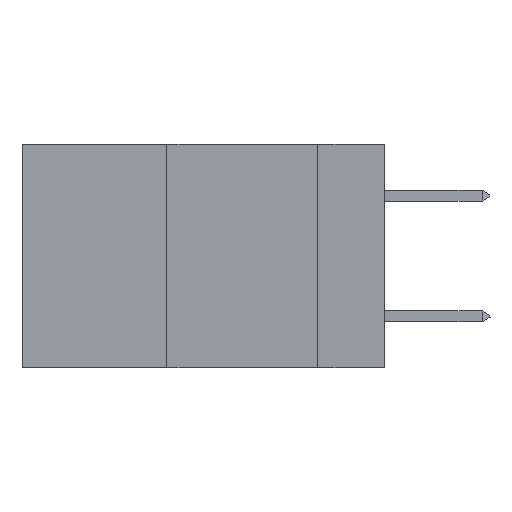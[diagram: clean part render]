
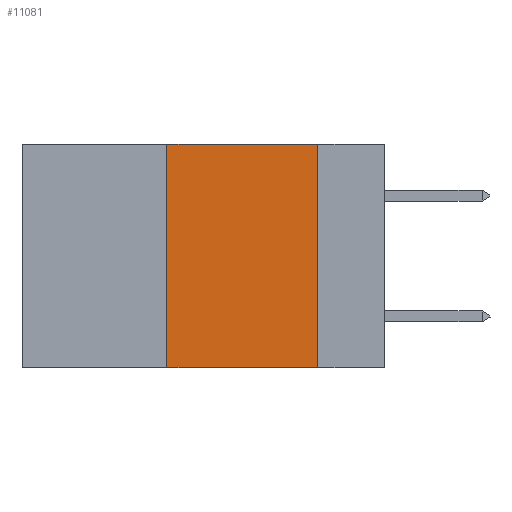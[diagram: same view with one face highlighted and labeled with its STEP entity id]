
A CAD part, left-side view. The second image highlights one B-rep face of the part: STEP entity #11081.
In plain terms, the highlighted planar face has unit normal (-1, 0, 0).
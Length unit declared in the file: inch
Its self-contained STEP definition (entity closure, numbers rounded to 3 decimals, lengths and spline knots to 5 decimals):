
#957 = DIRECTION ( 'NONE',  ( 0., 0., -1. ) ) ;
#1216 = EDGE_LOOP ( 'NONE', ( #5683, #15157, #14029, #14795 ) ) ;
#2191 = VECTOR ( 'NONE', #5154, 39.37008 ) ;
#2576 = CARTESIAN_POINT ( 'NONE',  ( 0., 0.36, 0. ) ) ;
#3693 = EDGE_CURVE ( 'NONE', #4525, #5397, #11834, .T. ) ;
#3724 = CARTESIAN_POINT ( 'NONE',  ( 0., 0.11, -0.37 ) ) ;
#4525 = VERTEX_POINT ( 'NONE', #11660 ) ;
#5057 = EDGE_CURVE ( 'NONE', #7020, #4525, #5782, .T. ) ;
#5154 = DIRECTION ( 'NONE',  ( 0., -1., 0. ) ) ;
#5188 = DIRECTION ( 'NONE',  ( 0., 0., -1. ) ) ;
#5397 = VERTEX_POINT ( 'NONE', #7984 ) ;
#5683 = ORIENTED_EDGE ( 'NONE', *, *, #15193, .F. ) ;
#5745 = VERTEX_POINT ( 'NONE', #3724 ) ;
#5782 = LINE ( 'NONE', #2576, #12210 ) ;
#6328 = LINE ( 'NONE', #12430, #12754 ) ;
#6542 = LINE ( 'NONE', #11416, #11831 ) ;
#6991 = PLANE ( 'NONE',  #10068 ) ;
#7020 = VERTEX_POINT ( 'NONE', #15474 ) ;
#7984 = CARTESIAN_POINT ( 'NONE',  ( 0., 0.11, 0. ) ) ;
#8208 = DIRECTION ( 'NONE',  ( 1., 0., 0. ) ) ;
#9225 = FACE_OUTER_BOUND ( 'NONE', #1216, .T. ) ;
#10068 = AXIS2_PLACEMENT_3D ( 'NONE', #15449, #8208, #957 ) ;
#11046 = DIRECTION ( 'NONE',  ( 0., 0., 1. ) ) ;
#11081 = ADVANCED_FACE ( 'NONE', ( #9225 ), #6991, .F. ) ;
#11416 = CARTESIAN_POINT ( 'NONE',  ( 0., 0.6, -0.37 ) ) ;
#11660 = CARTESIAN_POINT ( 'NONE',  ( 0., 0.36, 0. ) ) ;
#11831 = VECTOR ( 'NONE', #12615, 39.37008 ) ;
#11834 = LINE ( 'NONE', #13589, #2191 ) ;
#12210 = VECTOR ( 'NONE', #11046, 39.37008 ) ;
#12430 = CARTESIAN_POINT ( 'NONE',  ( 0., 0.11, 0. ) ) ;
#12615 = DIRECTION ( 'NONE',  ( 0., -1., 0. ) ) ;
#12754 = VECTOR ( 'NONE', #5188, 39.37008 ) ;
#13589 = CARTESIAN_POINT ( 'NONE',  ( 0., 0.6, 0. ) ) ;
#14029 = ORIENTED_EDGE ( 'NONE', *, *, #5057, .F. ) ;
#14630 = EDGE_CURVE ( 'NONE', #7020, #5745, #6542, .T. ) ;
#14795 = ORIENTED_EDGE ( 'NONE', *, *, #14630, .T. ) ;
#15157 = ORIENTED_EDGE ( 'NONE', *, *, #3693, .F. ) ;
#15193 = EDGE_CURVE ( 'NONE', #5397, #5745, #6328, .T. ) ;
#15449 = CARTESIAN_POINT ( 'NONE',  ( 0., 0.6, 0. ) ) ;
#15474 = CARTESIAN_POINT ( 'NONE',  ( 0., 0.36, -0.37 ) ) ;
